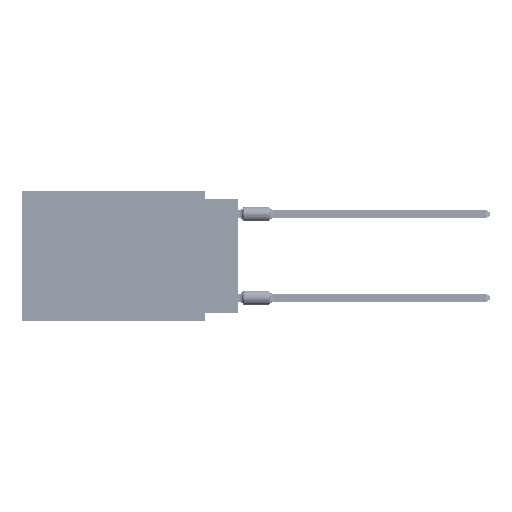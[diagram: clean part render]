
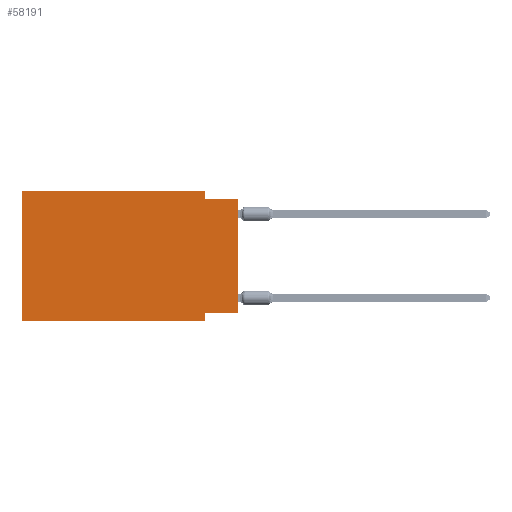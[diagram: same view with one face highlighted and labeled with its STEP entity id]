
A CAD part, left-side view. The second image highlights one B-rep face of the part: STEP entity #58191.
In plain terms, the highlighted planar face has unit normal (-1, 0, 0).
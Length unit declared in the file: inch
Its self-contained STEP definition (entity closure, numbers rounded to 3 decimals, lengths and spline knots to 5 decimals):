
#943 = DIRECTION ( 'NONE',  ( 0., 0., 1. ) ) ;
#1537 = DIRECTION ( 'NONE',  ( 0., -1., 0. ) ) ;
#2094 = EDGE_CURVE ( 'NONE', #25900, #20760, #13753, .T. ) ;
#2343 = VECTOR ( 'NONE', #24797, 39.37008 ) ;
#3003 = ORIENTED_EDGE ( 'NONE', *, *, #2094, .T. ) ;
#6161 = VECTOR ( 'NONE', #28012, 39.37008 ) ;
#8347 = CARTESIAN_POINT ( 'NONE',  ( 0., 0.1, -0.365 ) ) ;
#8789 = VECTOR ( 'NONE', #71017, 39.37008 ) ;
#9201 = LINE ( 'NONE', #9623, #6161 ) ;
#9335 = CARTESIAN_POINT ( 'NONE',  ( 0., 0.1, 0. ) ) ;
#9623 = CARTESIAN_POINT ( 'NONE',  ( 0., 0.1, 0. ) ) ;
#10608 = VECTOR ( 'NONE', #1537, 39.37008 ) ;
#13182 = ORIENTED_EDGE ( 'NONE', *, *, #71031, .F. ) ;
#13753 = LINE ( 'NONE', #79101, #26548 ) ;
#13768 = DIRECTION ( 'NONE',  ( 0., -1., 0. ) ) ;
#15129 = LINE ( 'NONE', #67264, #58240 ) ;
#16841 = ORIENTED_EDGE ( 'NONE', *, *, #28220, .F. ) ;
#17141 = LINE ( 'NONE', #17567, #2343 ) ;
#17567 = CARTESIAN_POINT ( 'NONE',  ( 0., 0.1, -0.39 ) ) ;
#18933 = EDGE_CURVE ( 'NONE', #46931, #20409, #79760, .T. ) ;
#20409 = VERTEX_POINT ( 'NONE', #43270 ) ;
#20536 = CARTESIAN_POINT ( 'NONE',  ( 0., 0.645, -0.39 ) ) ;
#20760 = VERTEX_POINT ( 'NONE', #60615 ) ;
#21243 = CARTESIAN_POINT ( 'NONE',  ( 0., 0.645, -0.39 ) ) ;
#22900 = CARTESIAN_POINT ( 'NONE',  ( 0., 0.1, -0.025 ) ) ;
#23262 = EDGE_LOOP ( 'NONE', ( #3003, #32134, #34902, #13182, #78810, #28760, #65803, #16841 ) ) ;
#24797 = DIRECTION ( 'NONE',  ( 0., 0., -1. ) ) ;
#25208 = EDGE_CURVE ( 'NONE', #46931, #33686, #52225, .T. ) ;
#25900 = VERTEX_POINT ( 'NONE', #42244 ) ;
#26454 = EDGE_CURVE ( 'NONE', #33259, #20760, #26577, .T. ) ;
#26548 = VECTOR ( 'NONE', #943, 39.37008 ) ;
#26577 = LINE ( 'NONE', #46239, #82579 ) ;
#28012 = DIRECTION ( 'NONE',  ( 0., 0., -1. ) ) ;
#28066 = DIRECTION ( 'NONE',  ( 0., -1., 0. ) ) ;
#28220 = EDGE_CURVE ( 'NONE', #25900, #65474, #15129, .T. ) ;
#28665 = EDGE_CURVE ( 'NONE', #65474, #20409, #17141, .T. ) ;
#28760 = ORIENTED_EDGE ( 'NONE', *, *, #18933, .T. ) ;
#32134 = ORIENTED_EDGE ( 'NONE', *, *, #26454, .F. ) ;
#33259 = VERTEX_POINT ( 'NONE', #22900 ) ;
#33686 = VERTEX_POINT ( 'NONE', #36886 ) ;
#34902 = ORIENTED_EDGE ( 'NONE', *, *, #35644, .F. ) ;
#35644 = EDGE_CURVE ( 'NONE', #49847, #33259, #9201, .T. ) ;
#36691 = CARTESIAN_POINT ( 'NONE',  ( 0., 0.645, 0. ) ) ;
#36886 = CARTESIAN_POINT ( 'NONE',  ( 0., 0.645, 0. ) ) ;
#40830 = LINE ( 'NONE', #74143, #10608 ) ;
#42244 = CARTESIAN_POINT ( 'NONE',  ( 0., 0., -0.365 ) ) ;
#43270 = CARTESIAN_POINT ( 'NONE',  ( 0., 0.1, -0.39 ) ) ;
#43508 = DIRECTION ( 'NONE',  ( 0., 0., -1. ) ) ;
#43932 = DIRECTION ( 'NONE',  ( 1., 0., 0. ) ) ;
#44342 = PLANE ( 'NONE',  #70521 ) ;
#44960 = CARTESIAN_POINT ( 'NONE',  ( 0., 0.645, 0. ) ) ;
#46239 = CARTESIAN_POINT ( 'NONE',  ( 0., 0., -0.025 ) ) ;
#46931 = VERTEX_POINT ( 'NONE', #20536 ) ;
#49847 = VERTEX_POINT ( 'NONE', #9335 ) ;
#50619 = VECTOR ( 'NONE', #28066, 39.37008 ) ;
#52225 = LINE ( 'NONE', #44960, #8789 ) ;
#56326 = FACE_OUTER_BOUND ( 'NONE', #23262, .T. ) ;
#58191 = ADVANCED_FACE ( 'NONE', ( #56326 ), #44342, .F. ) ;
#58240 = VECTOR ( 'NONE', #67671, 39.37008 ) ;
#60615 = CARTESIAN_POINT ( 'NONE',  ( 0., 0., -0.025 ) ) ;
#65474 = VERTEX_POINT ( 'NONE', #8347 ) ;
#65803 = ORIENTED_EDGE ( 'NONE', *, *, #28665, .F. ) ;
#67264 = CARTESIAN_POINT ( 'NONE',  ( 0., 0., -0.365 ) ) ;
#67671 = DIRECTION ( 'NONE',  ( 0., 1., 0. ) ) ;
#70521 = AXIS2_PLACEMENT_3D ( 'NONE', #36691, #43932, #43508 ) ;
#71017 = DIRECTION ( 'NONE',  ( 0., 0., 1. ) ) ;
#71031 = EDGE_CURVE ( 'NONE', #33686, #49847, #40830, .T. ) ;
#74143 = CARTESIAN_POINT ( 'NONE',  ( 0., 0.645, 0. ) ) ;
#78810 = ORIENTED_EDGE ( 'NONE', *, *, #25208, .F. ) ;
#79101 = CARTESIAN_POINT ( 'NONE',  ( 0., 0., 0. ) ) ;
#79760 = LINE ( 'NONE', #21243, #50619 ) ;
#82579 = VECTOR ( 'NONE', #13768, 39.37008 ) ;
